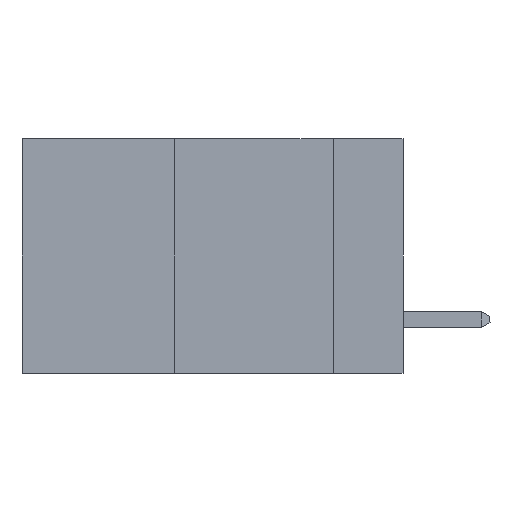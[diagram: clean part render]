
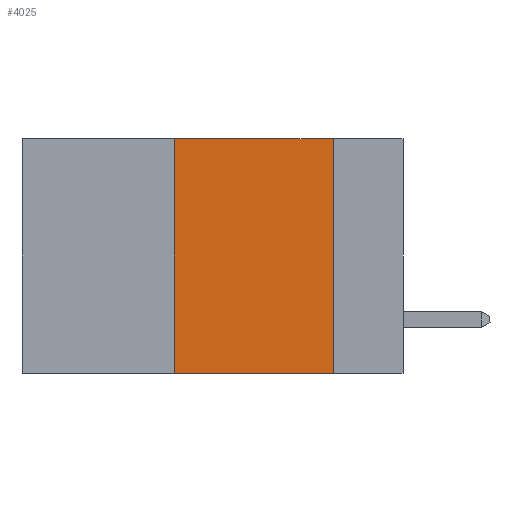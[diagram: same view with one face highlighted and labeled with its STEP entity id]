
A CAD part, left-side view. The second image highlights one B-rep face of the part: STEP entity #4025.
In plain terms, the highlighted planar face has unit normal (-1, 0, 0).
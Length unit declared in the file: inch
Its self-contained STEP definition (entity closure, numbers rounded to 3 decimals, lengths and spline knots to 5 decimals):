
#196 = CARTESIAN_POINT ( 'NONE',  ( 0., 0.6, -0.37 ) ) ;
#225 = ORIENTED_EDGE ( 'NONE', *, *, #9765, .F. ) ;
#568 = EDGE_CURVE ( 'NONE', #7069, #11523, #14729, .T. ) ;
#672 = DIRECTION ( 'NONE',  ( 0., 0., 1. ) ) ;
#936 = LINE ( 'NONE', #4544, #13581 ) ;
#1059 = CARTESIAN_POINT ( 'NONE',  ( 0., 0.6, 0. ) ) ;
#1076 = AXIS2_PLACEMENT_3D ( 'NONE', #4103, #4044, #14881 ) ;
#2896 = PLANE ( 'NONE',  #1076 ) ;
#3863 = EDGE_LOOP ( 'NONE', ( #9245, #12539, #225, #5187 ) ) ;
#4025 = ADVANCED_FACE ( 'NONE', ( #7444 ), #2896, .F. ) ;
#4044 = DIRECTION ( 'NONE',  ( 1., 0., 0. ) ) ;
#4103 = CARTESIAN_POINT ( 'NONE',  ( 0., 0.6, 0. ) ) ;
#4544 = CARTESIAN_POINT ( 'NONE',  ( 0., 0.11, 0. ) ) ;
#5187 = ORIENTED_EDGE ( 'NONE', *, *, #9097, .T. ) ;
#7010 = VERTEX_POINT ( 'NONE', #10022 ) ;
#7069 = VERTEX_POINT ( 'NONE', #9258 ) ;
#7444 = FACE_OUTER_BOUND ( 'NONE', #3863, .T. ) ;
#8616 = DIRECTION ( 'NONE',  ( 0., -1., 0. ) ) ;
#9097 = EDGE_CURVE ( 'NONE', #11106, #7010, #13049, .T. ) ;
#9182 = DIRECTION ( 'NONE',  ( 0., 0., -1. ) ) ;
#9200 = VECTOR ( 'NONE', #14348, 39.37008 ) ;
#9245 = ORIENTED_EDGE ( 'NONE', *, *, #9300, .F. ) ;
#9258 = CARTESIAN_POINT ( 'NONE',  ( 0., 0.36, 0. ) ) ;
#9300 = EDGE_CURVE ( 'NONE', #11523, #7010, #936, .T. ) ;
#9569 = VECTOR ( 'NONE', #672, 39.37008 ) ;
#9765 = EDGE_CURVE ( 'NONE', #11106, #7069, #14738, .T. ) ;
#10022 = CARTESIAN_POINT ( 'NONE',  ( 0., 0.11, -0.37 ) ) ;
#11106 = VERTEX_POINT ( 'NONE', #12743 ) ;
#11523 = VERTEX_POINT ( 'NONE', #14144 ) ;
#11538 = CARTESIAN_POINT ( 'NONE',  ( 0., 0.36, 0. ) ) ;
#12539 = ORIENTED_EDGE ( 'NONE', *, *, #568, .F. ) ;
#12743 = CARTESIAN_POINT ( 'NONE',  ( 0., 0.36, -0.37 ) ) ;
#13049 = LINE ( 'NONE', #196, #13230 ) ;
#13230 = VECTOR ( 'NONE', #8616, 39.37008 ) ;
#13581 = VECTOR ( 'NONE', #9182, 39.37008 ) ;
#14144 = CARTESIAN_POINT ( 'NONE',  ( 0., 0.11, 0. ) ) ;
#14348 = DIRECTION ( 'NONE',  ( 0., -1., 0. ) ) ;
#14729 = LINE ( 'NONE', #1059, #9200 ) ;
#14738 = LINE ( 'NONE', #11538, #9569 ) ;
#14881 = DIRECTION ( 'NONE',  ( 0., 0., -1. ) ) ;
